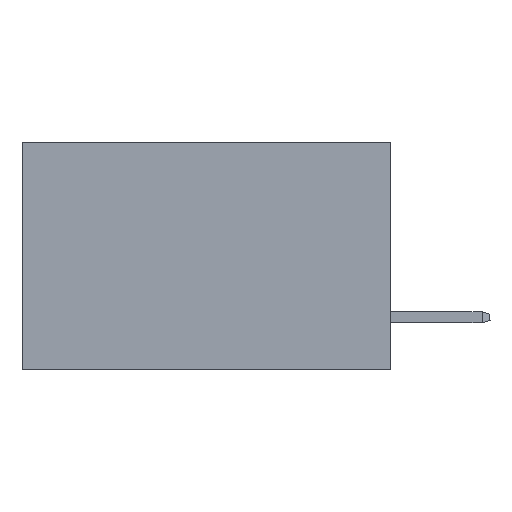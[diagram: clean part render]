
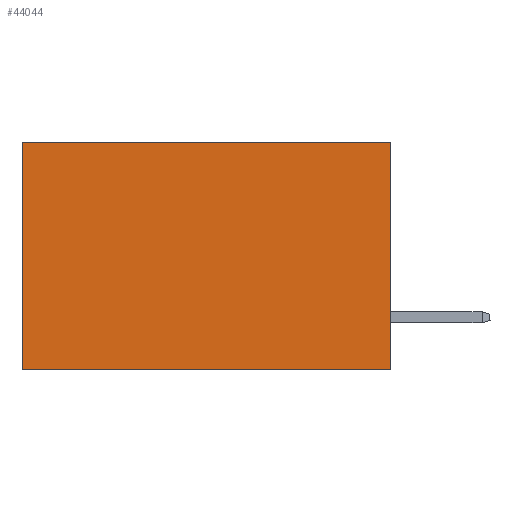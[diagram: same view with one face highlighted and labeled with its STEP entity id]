
A CAD part, left-side view. The second image highlights one B-rep face of the part: STEP entity #44044.
In plain terms, the highlighted planar face has unit normal (-1, 0, 0).
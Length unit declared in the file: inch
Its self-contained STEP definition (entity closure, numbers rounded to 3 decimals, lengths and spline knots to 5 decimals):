
#54 = FACE_OUTER_BOUND ( 'NONE', #41055, .T. ) ;
#197 = VECTOR ( 'NONE', #17110, 39.37008 ) ;
#257 = AXIS2_PLACEMENT_3D ( 'NONE', #1716, #29651, #8985 ) ;
#1716 = CARTESIAN_POINT ( 'NONE',  ( 0.2875, 0., 0. ) ) ;
#3944 = CARTESIAN_POINT ( 'NONE',  ( 0.2875, 0., -0.37 ) ) ;
#6034 = VECTOR ( 'NONE', #7120, 39.37008 ) ;
#6243 = ORIENTED_EDGE ( 'NONE', *, *, #18687, .F. ) ;
#6460 = CARTESIAN_POINT ( 'NONE',  ( 0.2875, 0.6, 0. ) ) ;
#7120 = DIRECTION ( 'NONE',  ( 0., 1., 0. ) ) ;
#7485 = DIRECTION ( 'NONE',  ( 0., 0., -1. ) ) ;
#8985 = DIRECTION ( 'NONE',  ( 0., 0., -1. ) ) ;
#9428 = LINE ( 'NONE', #44563, #197 ) ;
#11762 = EDGE_CURVE ( 'NONE', #18836, #37398, #25566, .T. ) ;
#12853 = CARTESIAN_POINT ( 'NONE',  ( 0.2875, 0., 0. ) ) ;
#14417 = CARTESIAN_POINT ( 'NONE',  ( 0.2875, 0.6, 0. ) ) ;
#17110 = DIRECTION ( 'NONE',  ( 0., 1., 0. ) ) ;
#17458 = CARTESIAN_POINT ( 'NONE',  ( 0.2875, 0., 0. ) ) ;
#18687 = EDGE_CURVE ( 'NONE', #19786, #20644, #20007, .T. ) ;
#18836 = VERTEX_POINT ( 'NONE', #14417 ) ;
#18910 = VECTOR ( 'NONE', #41710, 39.37008 ) ;
#19786 = VERTEX_POINT ( 'NONE', #12853 ) ;
#20007 = LINE ( 'NONE', #17458, #18910 ) ;
#20413 = CARTESIAN_POINT ( 'NONE',  ( 0.2875, 0., -0.37 ) ) ;
#20644 = VERTEX_POINT ( 'NONE', #20413 ) ;
#23813 = ORIENTED_EDGE ( 'NONE', *, *, #34314, .T. ) ;
#25566 = LINE ( 'NONE', #6460, #26113 ) ;
#26113 = VECTOR ( 'NONE', #7485, 39.37008 ) ;
#29651 = DIRECTION ( 'NONE',  ( 1., 0., 0. ) ) ;
#34314 = EDGE_CURVE ( 'NONE', #19786, #18836, #9428, .T. ) ;
#35750 = EDGE_CURVE ( 'NONE', #20644, #37398, #41334, .T. ) ;
#37398 = VERTEX_POINT ( 'NONE', #37685 ) ;
#37685 = CARTESIAN_POINT ( 'NONE',  ( 0.2875, 0.6, -0.37 ) ) ;
#38342 = ORIENTED_EDGE ( 'NONE', *, *, #35750, .F. ) ;
#41055 = EDGE_LOOP ( 'NONE', ( #42339, #38342, #6243, #23813 ) ) ;
#41334 = LINE ( 'NONE', #3944, #6034 ) ;
#41710 = DIRECTION ( 'NONE',  ( 0., 0., -1. ) ) ;
#42339 = ORIENTED_EDGE ( 'NONE', *, *, #11762, .T. ) ;
#43264 = PLANE ( 'NONE',  #257 ) ;
#44044 = ADVANCED_FACE ( 'NONE', ( #54 ), #43264, .F. ) ;
#44563 = CARTESIAN_POINT ( 'NONE',  ( 0.2875, 0., 0. ) ) ;
